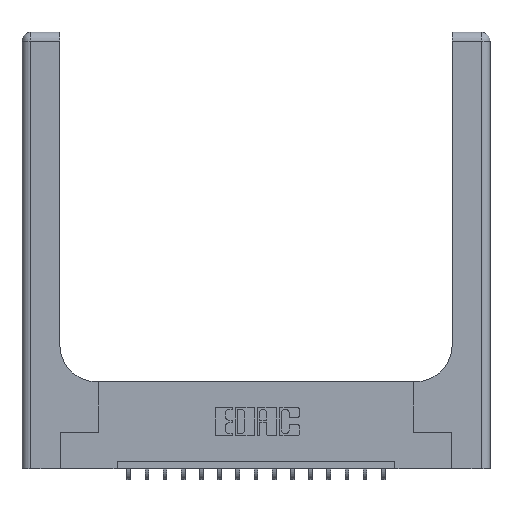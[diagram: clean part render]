
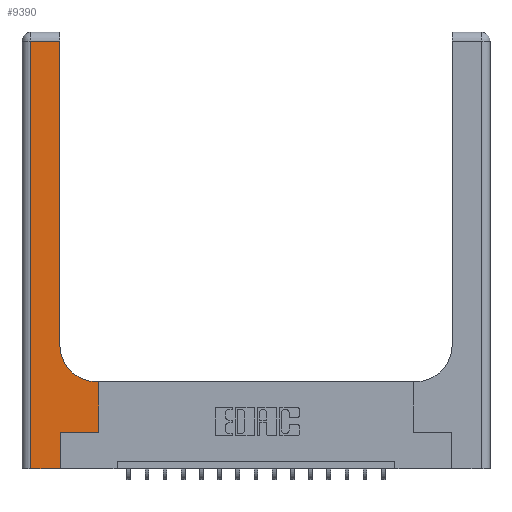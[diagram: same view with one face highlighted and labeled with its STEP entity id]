
A CAD part, top view. The second image highlights one B-rep face of the part: STEP entity #9390.
In plain terms, the highlighted planar face has unit normal (0, 0, 1).
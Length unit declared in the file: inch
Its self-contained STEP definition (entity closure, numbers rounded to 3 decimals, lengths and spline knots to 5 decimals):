
#97 = ORIENTED_EDGE ( 'NONE', *, *, #11007, .T. ) ;
#288 = ORIENTED_EDGE ( 'NONE', *, *, #3991, .T. ) ;
#321 = CARTESIAN_POINT ( 'NONE',  ( 0.265, 0., 0.37 ) ) ;
#369 = CARTESIAN_POINT ( 'NONE',  ( 0.528, 0.25, 0.37 ) ) ;
#563 = ORIENTED_EDGE ( 'NONE', *, *, #3586, .T. ) ;
#1031 = VECTOR ( 'NONE', #17842, 39.37008 ) ;
#1071 = CARTESIAN_POINT ( 'NONE',  ( 0.06, 0., 0.37 ) ) ;
#1467 = EDGE_CURVE ( 'NONE', #2026, #7434, #16524, .T. ) ;
#2026 = VERTEX_POINT ( 'NONE', #6631 ) ;
#2182 = PLANE ( 'NONE',  #11131 ) ;
#2223 = EDGE_CURVE ( 'NONE', #8698, #11132, #17324, .T. ) ;
#2245 = EDGE_CURVE ( 'NONE', #13480, #10455, #3127, .T. ) ;
#2301 = VECTOR ( 'NONE', #17502, 39.37008 ) ;
#2334 = ORIENTED_EDGE ( 'NONE', *, *, #11632, .T. ) ;
#2467 = CARTESIAN_POINT ( 'NONE',  ( 0., 3., 0.37 ) ) ;
#2546 = VECTOR ( 'NONE', #10077, 39.37008 ) ;
#2933 = LINE ( 'NONE', #10039, #8945 ) ;
#2941 = DIRECTION ( 'NONE',  ( 0., 1., 0. ) ) ;
#3000 = ORIENTED_EDGE ( 'NONE', *, *, #2223, .T. ) ;
#3012 = ORIENTED_EDGE ( 'NONE', *, *, #2245, .T. ) ;
#3127 = LINE ( 'NONE', #11681, #2301 ) ;
#3586 = EDGE_CURVE ( 'NONE', #11132, #4797, #7132, .T. ) ;
#3600 = EDGE_CURVE ( 'NONE', #4274, #8145, #17252, .T. ) ;
#3648 = CIRCLE ( 'NONE', #10019, 0.25 ) ;
#3669 = ORIENTED_EDGE ( 'NONE', *, *, #1467, .T. ) ;
#3991 = EDGE_CURVE ( 'NONE', #8145, #8698, #2933, .T. ) ;
#4008 = CARTESIAN_POINT ( 'NONE',  ( 0.26, 2.94, 0.37 ) ) ;
#4274 = VERTEX_POINT ( 'NONE', #5744 ) ;
#4797 = VERTEX_POINT ( 'NONE', #369 ) ;
#4978 = EDGE_CURVE ( 'NONE', #10455, #2026, #3648, .T. ) ;
#5100 = DIRECTION ( 'NONE',  ( 0., 0., -1. ) ) ;
#5104 = DIRECTION ( 'NONE',  ( -1., 0., 0. ) ) ;
#5558 = VECTOR ( 'NONE', #18465, 39.37008 ) ;
#5646 = CARTESIAN_POINT ( 'NONE',  ( 0.528, 0.25, 0.37 ) ) ;
#5707 = CARTESIAN_POINT ( 'NONE',  ( 0.06, 3., 0.37 ) ) ;
#5744 = CARTESIAN_POINT ( 'NONE',  ( 0.06, 2.94, 0.37 ) ) ;
#5877 = DIRECTION ( 'NONE',  ( 1., 0., 0. ) ) ;
#6309 = VECTOR ( 'NONE', #14642, 39.37008 ) ;
#6311 = CARTESIAN_POINT ( 'NONE',  ( 0.26, 3., 0.37 ) ) ;
#6631 = CARTESIAN_POINT ( 'NONE',  ( 0.26, 0.85, 0.37 ) ) ;
#7132 = LINE ( 'NONE', #10178, #5558 ) ;
#7434 = VERTEX_POINT ( 'NONE', #4008 ) ;
#7838 = VECTOR ( 'NONE', #5104, 39.37008 ) ;
#8145 = VERTEX_POINT ( 'NONE', #1071 ) ;
#8698 = VERTEX_POINT ( 'NONE', #8766 ) ;
#8766 = CARTESIAN_POINT ( 'NONE',  ( 0.265, 0., 0.37 ) ) ;
#8945 = VECTOR ( 'NONE', #5877, 39.37008 ) ;
#9390 = ADVANCED_FACE ( 'NONE', ( #13924 ), #2182, .F. ) ;
#9422 = CARTESIAN_POINT ( 'NONE',  ( 0.51, 0.85, 0.37 ) ) ;
#10019 = AXIS2_PLACEMENT_3D ( 'NONE', #9422, #13961, #16970 ) ;
#10039 = CARTESIAN_POINT ( 'NONE',  ( 0., 0., 0.37 ) ) ;
#10077 = DIRECTION ( 'NONE',  ( 0., -1., 0. ) ) ;
#10178 = CARTESIAN_POINT ( 'NONE',  ( 0.265, 0.25, 0.37 ) ) ;
#10218 = ORIENTED_EDGE ( 'NONE', *, *, #4978, .T. ) ;
#10455 = VERTEX_POINT ( 'NONE', #18427 ) ;
#11007 = EDGE_CURVE ( 'NONE', #4797, #13480, #14267, .T. ) ;
#11131 = AXIS2_PLACEMENT_3D ( 'NONE', #2467, #5100, #16931 ) ;
#11132 = VERTEX_POINT ( 'NONE', #12929 ) ;
#11632 = EDGE_CURVE ( 'NONE', #7434, #4274, #13834, .T. ) ;
#11681 = CARTESIAN_POINT ( 'NONE',  ( 0.26, 0.6, 0.37 ) ) ;
#12929 = CARTESIAN_POINT ( 'NONE',  ( 0.265, 0.25, 0.37 ) ) ;
#13480 = VERTEX_POINT ( 'NONE', #18499 ) ;
#13834 = LINE ( 'NONE', #16757, #7838 ) ;
#13924 = FACE_OUTER_BOUND ( 'NONE', #15341, .T. ) ;
#13961 = DIRECTION ( 'NONE',  ( 0., 0., -1. ) ) ;
#14267 = LINE ( 'NONE', #5646, #6309 ) ;
#14379 = VECTOR ( 'NONE', #2941, 39.37008 ) ;
#14642 = DIRECTION ( 'NONE',  ( 0., 1., 0. ) ) ;
#15341 = EDGE_LOOP ( 'NONE', ( #3669, #2334, #16082, #288, #3000, #563, #97, #3012, #10218 ) ) ;
#16082 = ORIENTED_EDGE ( 'NONE', *, *, #3600, .T. ) ;
#16524 = LINE ( 'NONE', #6311, #1031 ) ;
#16757 = CARTESIAN_POINT ( 'NONE',  ( 0., 2.94, 0.37 ) ) ;
#16931 = DIRECTION ( 'NONE',  ( -1., 0., 0. ) ) ;
#16970 = DIRECTION ( 'NONE',  ( 1., 0., 0. ) ) ;
#17252 = LINE ( 'NONE', #5707, #2546 ) ;
#17324 = LINE ( 'NONE', #321, #14379 ) ;
#17502 = DIRECTION ( 'NONE',  ( -1., 0., 0. ) ) ;
#17842 = DIRECTION ( 'NONE',  ( 0., 1., 0. ) ) ;
#18427 = CARTESIAN_POINT ( 'NONE',  ( 0.51, 0.6, 0.37 ) ) ;
#18465 = DIRECTION ( 'NONE',  ( 1., 0., 0. ) ) ;
#18499 = CARTESIAN_POINT ( 'NONE',  ( 0.528, 0.6, 0.37 ) ) ;
